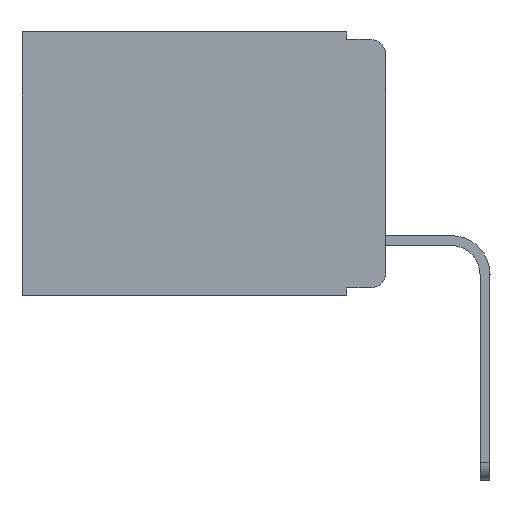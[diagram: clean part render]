
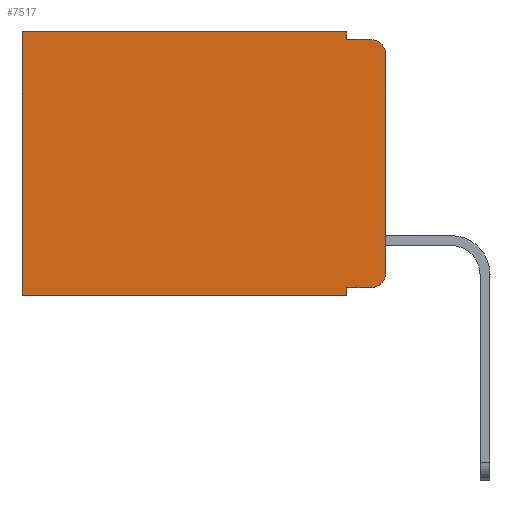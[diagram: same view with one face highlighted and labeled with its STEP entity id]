
A CAD part, left-side view. The second image highlights one B-rep face of the part: STEP entity #7517.
In plain terms, the highlighted planar face has unit normal (-1, 0, 0).
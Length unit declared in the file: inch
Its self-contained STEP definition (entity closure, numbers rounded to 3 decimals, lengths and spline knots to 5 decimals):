
#9 = VECTOR ( 'NONE', #2869, 39.37008 ) ;
#346 = CARTESIAN_POINT ( 'NONE',  ( 0.298, 0.02, -0.313 ) ) ;
#368 = VERTEX_POINT ( 'NONE', #15060 ) ;
#482 = CARTESIAN_POINT ( 'NONE',  ( 0.298, 0., 0. ) ) ;
#682 = CARTESIAN_POINT ( 'NONE',  ( 0.298, 0.051, -0.333 ) ) ;
#1011 = DIRECTION ( 'NONE',  ( -1., 0., 0. ) ) ;
#1073 = DIRECTION ( 'NONE',  ( 0., 0., -1. ) ) ;
#1437 = CARTESIAN_POINT ( 'NONE',  ( 0.298, 0.051, -0.01 ) ) ;
#1649 = VERTEX_POINT ( 'NONE', #12923 ) ;
#1746 = VECTOR ( 'NONE', #11467, 39.37008 ) ;
#2128 = DIRECTION ( 'NONE',  ( 0., 0., -1. ) ) ;
#2261 = DIRECTION ( 'NONE',  ( 0., 0., -1. ) ) ;
#2315 = DIRECTION ( 'NONE',  ( 0., -1., 0. ) ) ;
#2869 = DIRECTION ( 'NONE',  ( 0., 0., -1. ) ) ;
#2920 = ORIENTED_EDGE ( 'NONE', *, *, #9782, .T. ) ;
#3122 = CARTESIAN_POINT ( 'NONE',  ( 0.298, 0., -0.03 ) ) ;
#3652 = VERTEX_POINT ( 'NONE', #18239 ) ;
#3830 = VECTOR ( 'NONE', #2261, 39.37008 ) ;
#4036 = EDGE_CURVE ( 'NONE', #1649, #4070, #7474, .T. ) ;
#4070 = VERTEX_POINT ( 'NONE', #11582 ) ;
#4217 = VECTOR ( 'NONE', #13453, 39.37008 ) ;
#4390 = AXIS2_PLACEMENT_3D ( 'NONE', #346, #7575, #6345 ) ;
#4406 = ORIENTED_EDGE ( 'NONE', *, *, #10529, .T. ) ;
#4518 = VERTEX_POINT ( 'NONE', #5982 ) ;
#5102 = DIRECTION ( 'NONE',  ( 0., 1., 0. ) ) ;
#5741 = EDGE_CURVE ( 'NONE', #18172, #8493, #9719, .T. ) ;
#5838 = EDGE_CURVE ( 'NONE', #11108, #3652, #18194, .T. ) ;
#5945 = ORIENTED_EDGE ( 'NONE', *, *, #11059, .F. ) ;
#5982 = CARTESIAN_POINT ( 'NONE',  ( 0.298, 0.051, 0. ) ) ;
#5984 = AXIS2_PLACEMENT_3D ( 'NONE', #12698, #1011, #1073 ) ;
#6110 = CARTESIAN_POINT ( 'NONE',  ( 0.298, 0.473, 0. ) ) ;
#6345 = DIRECTION ( 'NONE',  ( 0., 0., -1. ) ) ;
#6489 = DIRECTION ( 'NONE',  ( 0., 0., -1. ) ) ;
#6739 = CARTESIAN_POINT ( 'NONE',  ( 0.298, 0.051, 0. ) ) ;
#6998 = ORIENTED_EDGE ( 'NONE', *, *, #5838, .T. ) ;
#7429 = VECTOR ( 'NONE', #5102, 39.37008 ) ;
#7474 = LINE ( 'NONE', #1437, #1746 ) ;
#7517 = ADVANCED_FACE ( 'NONE', ( #8252 ), #13831, .F. ) ;
#7575 = DIRECTION ( 'NONE',  ( -1., 0., 0. ) ) ;
#8183 = LINE ( 'NONE', #6739, #3830 ) ;
#8252 = FACE_OUTER_BOUND ( 'NONE', #18462, .T. ) ;
#8493 = VERTEX_POINT ( 'NONE', #17859 ) ;
#8969 = ORIENTED_EDGE ( 'NONE', *, *, #18064, .F. ) ;
#9635 = CARTESIAN_POINT ( 'NONE',  ( 0.298, 0.051, -0.333 ) ) ;
#9719 = LINE ( 'NONE', #9635, #13360 ) ;
#9776 = CIRCLE ( 'NONE', #4390, 0.02 ) ;
#9782 = EDGE_CURVE ( 'NONE', #4518, #11108, #13268, .T. ) ;
#9927 = CARTESIAN_POINT ( 'NONE',  ( 0.298, 0., 0. ) ) ;
#9930 = EDGE_CURVE ( 'NONE', #18172, #368, #14635, .T. ) ;
#10223 = CARTESIAN_POINT ( 'NONE',  ( 0.298, 0., -0.313 ) ) ;
#10529 = EDGE_CURVE ( 'NONE', #13145, #4070, #18737, .T. ) ;
#10902 = CARTESIAN_POINT ( 'NONE',  ( 0.298, 0., 0. ) ) ;
#11059 = EDGE_CURVE ( 'NONE', #4518, #1649, #8183, .T. ) ;
#11108 = VERTEX_POINT ( 'NONE', #13901 ) ;
#11311 = LINE ( 'NONE', #13788, #7429 ) ;
#11384 = DIRECTION ( 'NONE',  ( 0., 1., 0. ) ) ;
#11437 = EDGE_CURVE ( 'NONE', #8493, #16832, #9776, .T. ) ;
#11467 = DIRECTION ( 'NONE',  ( 0., -1., 0. ) ) ;
#11582 = CARTESIAN_POINT ( 'NONE',  ( 0.298, 0.02, -0.01 ) ) ;
#12698 = CARTESIAN_POINT ( 'NONE',  ( 0.298, 0.02, -0.03 ) ) ;
#12889 = ORIENTED_EDGE ( 'NONE', *, *, #4036, .F. ) ;
#12907 = CARTESIAN_POINT ( 'NONE',  ( 0.298, 0.051, 0. ) ) ;
#12923 = CARTESIAN_POINT ( 'NONE',  ( 0.298, 0.051, -0.01 ) ) ;
#13145 = VERTEX_POINT ( 'NONE', #3122 ) ;
#13268 = LINE ( 'NONE', #9927, #15334 ) ;
#13290 = ORIENTED_EDGE ( 'NONE', *, *, #18666, .F. ) ;
#13360 = VECTOR ( 'NONE', #2315, 39.37008 ) ;
#13453 = DIRECTION ( 'NONE',  ( 0., 0., -1. ) ) ;
#13776 = DIRECTION ( 'NONE',  ( 1., 0., 0. ) ) ;
#13788 = CARTESIAN_POINT ( 'NONE',  ( 0.298, 0., -0.343 ) ) ;
#13831 = PLANE ( 'NONE',  #15249 ) ;
#13901 = CARTESIAN_POINT ( 'NONE',  ( 0.298, 0.473, 0. ) ) ;
#14177 = ORIENTED_EDGE ( 'NONE', *, *, #9930, .F. ) ;
#14485 = VECTOR ( 'NONE', #2128, 39.37008 ) ;
#14635 = LINE ( 'NONE', #12907, #9 ) ;
#15060 = CARTESIAN_POINT ( 'NONE',  ( 0.298, 0.051, -0.343 ) ) ;
#15189 = ORIENTED_EDGE ( 'NONE', *, *, #5741, .T. ) ;
#15249 = AXIS2_PLACEMENT_3D ( 'NONE', #482, #13776, #6489 ) ;
#15334 = VECTOR ( 'NONE', #11384, 39.37008 ) ;
#16105 = LINE ( 'NONE', #10902, #14485 ) ;
#16832 = VERTEX_POINT ( 'NONE', #10223 ) ;
#17859 = CARTESIAN_POINT ( 'NONE',  ( 0.298, 0.02, -0.333 ) ) ;
#18064 = EDGE_CURVE ( 'NONE', #368, #3652, #11311, .T. ) ;
#18087 = ORIENTED_EDGE ( 'NONE', *, *, #11437, .T. ) ;
#18172 = VERTEX_POINT ( 'NONE', #682 ) ;
#18194 = LINE ( 'NONE', #6110, #4217 ) ;
#18239 = CARTESIAN_POINT ( 'NONE',  ( 0.298, 0.473, -0.343 ) ) ;
#18462 = EDGE_LOOP ( 'NONE', ( #13290, #4406, #12889, #5945, #2920, #6998, #8969, #14177, #15189, #18087 ) ) ;
#18666 = EDGE_CURVE ( 'NONE', #13145, #16832, #16105, .T. ) ;
#18737 = CIRCLE ( 'NONE', #5984, 0.02 ) ;
